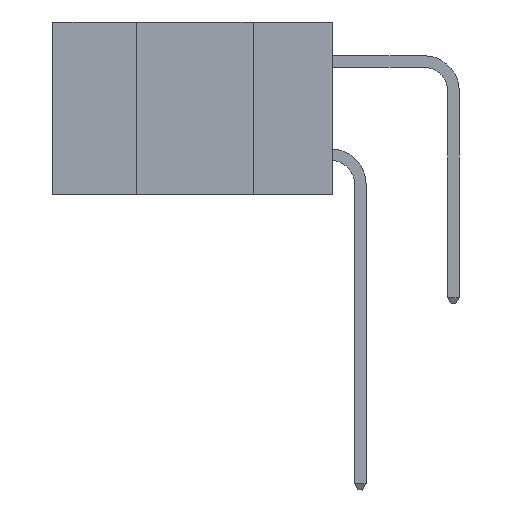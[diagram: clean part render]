
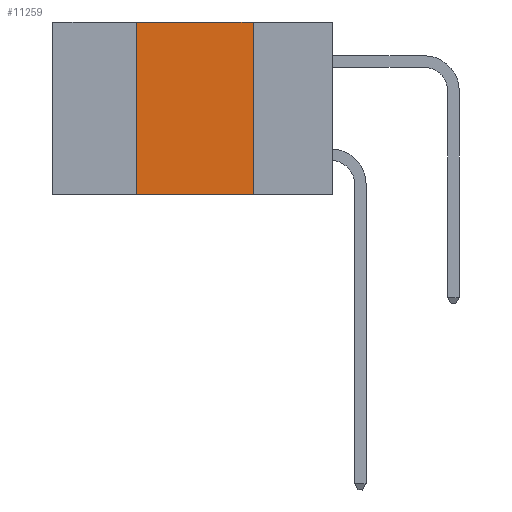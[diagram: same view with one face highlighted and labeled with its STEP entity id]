
A CAD part, left-side view. The second image highlights one B-rep face of the part: STEP entity #11259.
In plain terms, the highlighted planar face has unit normal (-1, 0, 0).
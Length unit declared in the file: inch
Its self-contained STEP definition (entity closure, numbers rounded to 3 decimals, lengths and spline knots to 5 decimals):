
#1354 = VERTEX_POINT ( 'NONE', #26863 ) ;
#1633 = CARTESIAN_POINT ( 'NONE',  ( 0., 0.17, -0.37 ) ) ;
#2109 = CARTESIAN_POINT ( 'NONE',  ( 0., 0.42, 0. ) ) ;
#2123 = CARTESIAN_POINT ( 'NONE',  ( 0., 0.6, 0. ) ) ;
#4608 = LINE ( 'NONE', #7473, #32695 ) ;
#4932 = DIRECTION ( 'NONE',  ( 0., 0., -1. ) ) ;
#5580 = ORIENTED_EDGE ( 'NONE', *, *, #7640, .F. ) ;
#6233 = CARTESIAN_POINT ( 'NONE',  ( 0., 0.6, -0.37 ) ) ;
#6470 = DIRECTION ( 'NONE',  ( 0., -1., 0. ) ) ;
#7473 = CARTESIAN_POINT ( 'NONE',  ( 0., 0.17, 0. ) ) ;
#7640 = EDGE_CURVE ( 'NONE', #15816, #8837, #4608, .T. ) ;
#8837 = VERTEX_POINT ( 'NONE', #1633 ) ;
#10523 = PLANE ( 'NONE',  #35005 ) ;
#11259 = ADVANCED_FACE ( 'NONE', ( #31188 ), #10523, .F. ) ;
#11499 = LINE ( 'NONE', #17708, #25539 ) ;
#12335 = EDGE_CURVE ( 'NONE', #1354, #15816, #11499, .T. ) ;
#14726 = LINE ( 'NONE', #2109, #29617 ) ;
#15816 = VERTEX_POINT ( 'NONE', #34394 ) ;
#16460 = VECTOR ( 'NONE', #23069, 39.37008 ) ;
#17101 = EDGE_CURVE ( 'NONE', #22106, #8837, #29579, .T. ) ;
#17708 = CARTESIAN_POINT ( 'NONE',  ( 0., 0.6, 0. ) ) ;
#18985 = EDGE_CURVE ( 'NONE', #22106, #1354, #14726, .T. ) ;
#21795 = DIRECTION ( 'NONE',  ( 1., 0., 0. ) ) ;
#21895 = EDGE_LOOP ( 'NONE', ( #5580, #30825, #26800, #31795 ) ) ;
#22106 = VERTEX_POINT ( 'NONE', #33728 ) ;
#23069 = DIRECTION ( 'NONE',  ( 0., -1., 0. ) ) ;
#24431 = DIRECTION ( 'NONE',  ( 0., 0., -1. ) ) ;
#25539 = VECTOR ( 'NONE', #6470, 39.37008 ) ;
#26800 = ORIENTED_EDGE ( 'NONE', *, *, #18985, .F. ) ;
#26863 = CARTESIAN_POINT ( 'NONE',  ( 0., 0.42, 0. ) ) ;
#29579 = LINE ( 'NONE', #6233, #16460 ) ;
#29617 = VECTOR ( 'NONE', #30088, 39.37008 ) ;
#30088 = DIRECTION ( 'NONE',  ( 0., 0., 1. ) ) ;
#30825 = ORIENTED_EDGE ( 'NONE', *, *, #12335, .F. ) ;
#31188 = FACE_OUTER_BOUND ( 'NONE', #21895, .T. ) ;
#31795 = ORIENTED_EDGE ( 'NONE', *, *, #17101, .T. ) ;
#32695 = VECTOR ( 'NONE', #24431, 39.37008 ) ;
#33728 = CARTESIAN_POINT ( 'NONE',  ( 0., 0.42, -0.37 ) ) ;
#34394 = CARTESIAN_POINT ( 'NONE',  ( 0., 0.17, 0. ) ) ;
#35005 = AXIS2_PLACEMENT_3D ( 'NONE', #2123, #21795, #4932 ) ;
